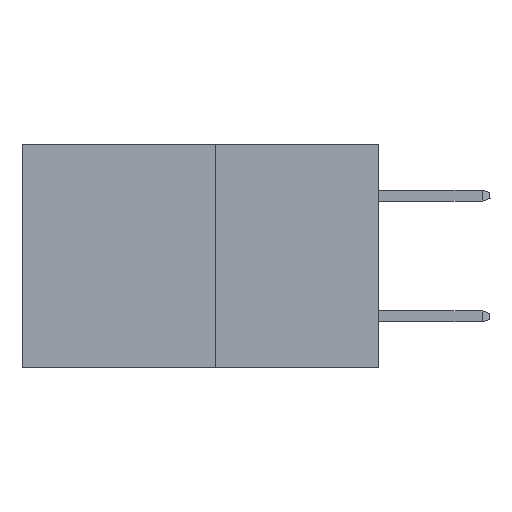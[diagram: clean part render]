
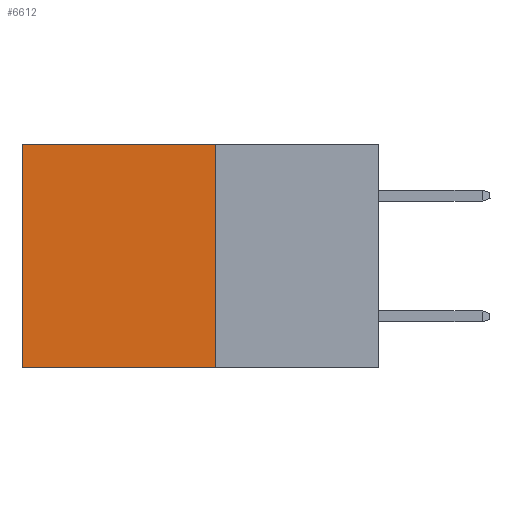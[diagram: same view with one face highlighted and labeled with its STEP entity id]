
A CAD part, left-side view. The second image highlights one B-rep face of the part: STEP entity #6612.
In plain terms, the highlighted planar face has unit normal (-1, 0, 0).
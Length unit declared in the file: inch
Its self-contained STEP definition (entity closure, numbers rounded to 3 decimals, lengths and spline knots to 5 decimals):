
#254 = VERTEX_POINT ( 'NONE', #4621 ) ;
#425 = LINE ( 'NONE', #6567, #2445 ) ;
#438 = VECTOR ( 'NONE', #5324, 39.37008 ) ;
#626 = ORIENTED_EDGE ( 'NONE', *, *, #4787, .T. ) ;
#907 = EDGE_CURVE ( 'NONE', #2105, #254, #7854, .T. ) ;
#1294 = FACE_OUTER_BOUND ( 'NONE', #2476, .T. ) ;
#1679 = CARTESIAN_POINT ( 'NONE',  ( 0.277, 0.27, -0.37 ) ) ;
#2105 = VERTEX_POINT ( 'NONE', #5180 ) ;
#2109 = DIRECTION ( 'NONE',  ( 0., 0., -1. ) ) ;
#2146 = DIRECTION ( 'NONE',  ( 0., 0., -1. ) ) ;
#2185 = VECTOR ( 'NONE', #9306, 39.37008 ) ;
#2445 = VECTOR ( 'NONE', #2109, 39.37008 ) ;
#2476 = EDGE_LOOP ( 'NONE', ( #3795, #9425, #6357, #626 ) ) ;
#2499 = VERTEX_POINT ( 'NONE', #8578 ) ;
#2505 = VERTEX_POINT ( 'NONE', #5009 ) ;
#3795 = ORIENTED_EDGE ( 'NONE', *, *, #7189, .T. ) ;
#3860 = EDGE_CURVE ( 'NONE', #2499, #2105, #4681, .T. ) ;
#4621 = CARTESIAN_POINT ( 'NONE',  ( 0.277, 0.59, -0.37 ) ) ;
#4681 = LINE ( 'NONE', #5053, #2185 ) ;
#4787 = EDGE_CURVE ( 'NONE', #2499, #2505, #9450, .T. ) ;
#4835 = CARTESIAN_POINT ( 'NONE',  ( 0.277, 0.27, 0. ) ) ;
#5009 = CARTESIAN_POINT ( 'NONE',  ( 0.277, 0.59, 0. ) ) ;
#5053 = CARTESIAN_POINT ( 'NONE',  ( 0.277, 0.27, -0.37 ) ) ;
#5180 = CARTESIAN_POINT ( 'NONE',  ( 0.277, 0.27, -0.37 ) ) ;
#5324 = DIRECTION ( 'NONE',  ( 0., 1., 0. ) ) ;
#5854 = AXIS2_PLACEMENT_3D ( 'NONE', #9377, #6615, #2146 ) ;
#5857 = PLANE ( 'NONE',  #5854 ) ;
#6357 = ORIENTED_EDGE ( 'NONE', *, *, #3860, .F. ) ;
#6567 = CARTESIAN_POINT ( 'NONE',  ( 0.277, 0.59, -0.37 ) ) ;
#6612 = ADVANCED_FACE ( 'NONE', ( #1294 ), #5857, .F. ) ;
#6615 = DIRECTION ( 'NONE',  ( 1., 0., 0. ) ) ;
#6999 = DIRECTION ( 'NONE',  ( 0., 1., 0. ) ) ;
#7189 = EDGE_CURVE ( 'NONE', #2505, #254, #425, .T. ) ;
#7593 = VECTOR ( 'NONE', #6999, 39.37008 ) ;
#7854 = LINE ( 'NONE', #1679, #438 ) ;
#8578 = CARTESIAN_POINT ( 'NONE',  ( 0.277, 0.27, 0. ) ) ;
#9306 = DIRECTION ( 'NONE',  ( 0., 0., -1. ) ) ;
#9377 = CARTESIAN_POINT ( 'NONE',  ( 0.277, 0.27, -0.37 ) ) ;
#9425 = ORIENTED_EDGE ( 'NONE', *, *, #907, .F. ) ;
#9450 = LINE ( 'NONE', #4835, #7593 ) ;
